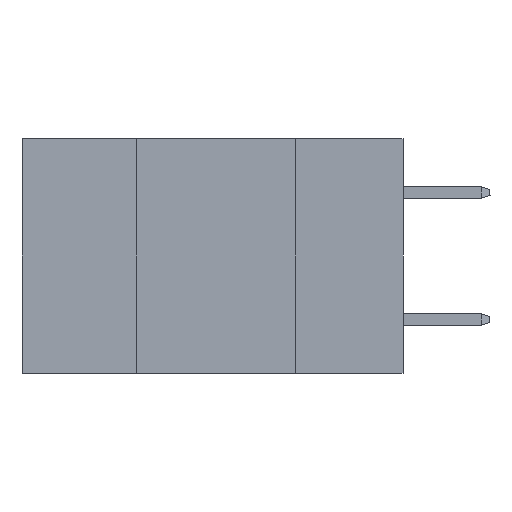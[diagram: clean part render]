
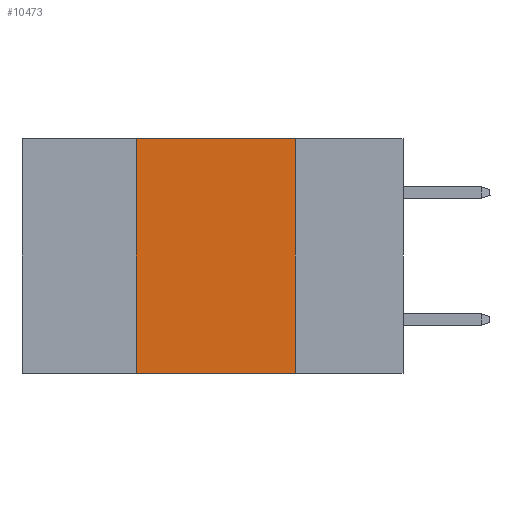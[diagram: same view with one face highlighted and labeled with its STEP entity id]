
A CAD part, left-side view. The second image highlights one B-rep face of the part: STEP entity #10473.
In plain terms, the highlighted planar face has unit normal (-1, 0, 0).
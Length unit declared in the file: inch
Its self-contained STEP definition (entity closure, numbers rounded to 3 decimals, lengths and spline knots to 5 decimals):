
#1056 = AXIS2_PLACEMENT_3D ( 'NONE', #21897, #25214, #22104 ) ;
#1812 = LINE ( 'NONE', #18360, #33175 ) ;
#2204 = VECTOR ( 'NONE', #23238, 39.37008 ) ;
#2736 = VECTOR ( 'NONE', #11945, 39.37008 ) ;
#3765 = EDGE_LOOP ( 'NONE', ( #36053, #18133, #7116, #23380 ) ) ;
#4161 = CARTESIAN_POINT ( 'NONE',  ( 0., 0.6, -0.37 ) ) ;
#4620 = LINE ( 'NONE', #7150, #36519 ) ;
#5207 = CARTESIAN_POINT ( 'NONE',  ( 0., 0.42, 0. ) ) ;
#7116 = ORIENTED_EDGE ( 'NONE', *, *, #24453, .F. ) ;
#7150 = CARTESIAN_POINT ( 'NONE',  ( 0., 0.6, 0. ) ) ;
#7531 = VERTEX_POINT ( 'NONE', #5207 ) ;
#10473 = ADVANCED_FACE ( 'NONE', ( #28103 ), #37710, .F. ) ;
#11945 = DIRECTION ( 'NONE',  ( 0., 0., 1. ) ) ;
#12141 = LINE ( 'NONE', #31441, #2736 ) ;
#13716 = EDGE_CURVE ( 'NONE', #22335, #18340, #1812, .T. ) ;
#18133 = ORIENTED_EDGE ( 'NONE', *, *, #25173, .F. ) ;
#18340 = VERTEX_POINT ( 'NONE', #37163 ) ;
#18360 = CARTESIAN_POINT ( 'NONE',  ( 0., 0.17, 0. ) ) ;
#18480 = CARTESIAN_POINT ( 'NONE',  ( 0., 0.17, 0. ) ) ;
#19470 = VERTEX_POINT ( 'NONE', #38836 ) ;
#20692 = DIRECTION ( 'NONE',  ( 0., 0., -1. ) ) ;
#21897 = CARTESIAN_POINT ( 'NONE',  ( 0., 0.6, 0. ) ) ;
#22104 = DIRECTION ( 'NONE',  ( 0., 0., -1. ) ) ;
#22335 = VERTEX_POINT ( 'NONE', #18480 ) ;
#23082 = DIRECTION ( 'NONE',  ( 0., -1., 0. ) ) ;
#23238 = DIRECTION ( 'NONE',  ( 0., -1., 0. ) ) ;
#23380 = ORIENTED_EDGE ( 'NONE', *, *, #36263, .T. ) ;
#24453 = EDGE_CURVE ( 'NONE', #19470, #7531, #12141, .T. ) ;
#25173 = EDGE_CURVE ( 'NONE', #7531, #22335, #4620, .T. ) ;
#25214 = DIRECTION ( 'NONE',  ( 1., 0., 0. ) ) ;
#28103 = FACE_OUTER_BOUND ( 'NONE', #3765, .T. ) ;
#31441 = CARTESIAN_POINT ( 'NONE',  ( 0., 0.42, 0. ) ) ;
#33175 = VECTOR ( 'NONE', #20692, 39.37008 ) ;
#36053 = ORIENTED_EDGE ( 'NONE', *, *, #13716, .F. ) ;
#36140 = LINE ( 'NONE', #4161, #2204 ) ;
#36263 = EDGE_CURVE ( 'NONE', #19470, #18340, #36140, .T. ) ;
#36519 = VECTOR ( 'NONE', #23082, 39.37008 ) ;
#37163 = CARTESIAN_POINT ( 'NONE',  ( 0., 0.17, -0.37 ) ) ;
#37710 = PLANE ( 'NONE',  #1056 ) ;
#38836 = CARTESIAN_POINT ( 'NONE',  ( 0., 0.42, -0.37 ) ) ;
